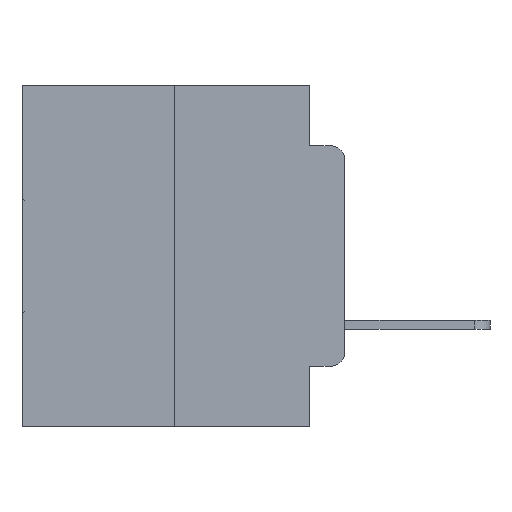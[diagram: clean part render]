
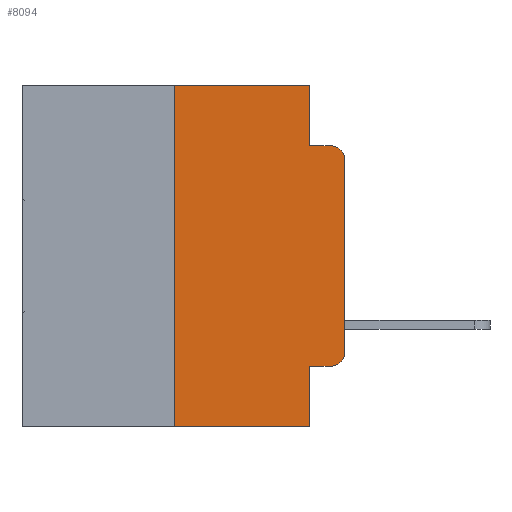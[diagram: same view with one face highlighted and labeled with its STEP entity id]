
A CAD part, left-side view. The second image highlights one B-rep face of the part: STEP entity #8094.
In plain terms, the highlighted planar face has unit normal (-1, 0, 0).
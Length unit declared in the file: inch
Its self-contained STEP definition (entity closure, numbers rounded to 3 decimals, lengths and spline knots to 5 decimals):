
#17 = ORIENTED_EDGE ( 'NONE', *, *, #22822, .F. ) ;
#304 = VERTEX_POINT ( 'NONE', #7070 ) ;
#640 = CARTESIAN_POINT ( 'NONE',  ( 0., 0.051, -0.4115 ) ) ;
#647 = ORIENTED_EDGE ( 'NONE', *, *, #26199, .F. ) ;
#725 = ORIENTED_EDGE ( 'NONE', *, *, #19845, .F. ) ;
#1121 = ORIENTED_EDGE ( 'NONE', *, *, #26100, .T. ) ;
#1159 = ORIENTED_EDGE ( 'NONE', *, *, #24348, .F. ) ;
#1205 = CARTESIAN_POINT ( 'NONE',  ( 0., 0.02, -0.3915 ) ) ;
#1344 = LINE ( 'NONE', #10655, #12297 ) ;
#1798 = DIRECTION ( 'NONE',  ( 0., 0., -1. ) ) ;
#2076 = ORIENTED_EDGE ( 'NONE', *, *, #5487, .T. ) ;
#2151 = CARTESIAN_POINT ( 'NONE',  ( 0., 0.25, 0. ) ) ;
#2738 = CARTESIAN_POINT ( 'NONE',  ( 0., 0.473, 0. ) ) ;
#2911 = EDGE_CURVE ( 'NONE', #21207, #26920, #1344, .T. ) ;
#3239 = ORIENTED_EDGE ( 'NONE', *, *, #10179, .T. ) ;
#3328 = DIRECTION ( 'NONE',  ( 0., -1., 0. ) ) ;
#3773 = DIRECTION ( 'NONE',  ( 0., 0., -1. ) ) ;
#5407 = DIRECTION ( 'NONE',  ( 0., -1., 0. ) ) ;
#5487 = EDGE_CURVE ( 'NONE', #23272, #24393, #9509, .T. ) ;
#6623 = LINE ( 'NONE', #21741, #19017 ) ;
#7070 = CARTESIAN_POINT ( 'NONE',  ( 0., 0.25, 0. ) ) ;
#7142 = ORIENTED_EDGE ( 'NONE', *, *, #21871, .F. ) ;
#8011 = VERTEX_POINT ( 'NONE', #21245 ) ;
#8057 = DIRECTION ( 'NONE',  ( 0., -1., 0. ) ) ;
#8094 = ADVANCED_FACE ( 'NONE', ( #28473 ), #26141, .F. ) ;
#8113 = EDGE_LOOP ( 'NONE', ( #11316, #24000, #7142, #17, #647, #725, #1121, #1159, #2076, #3239 ) ) ;
#8690 = CARTESIAN_POINT ( 'NONE',  ( 0., 0.051, 0. ) ) ;
#8902 = CARTESIAN_POINT ( 'NONE',  ( 0., 0.02, -0.4115 ) ) ;
#9316 = VECTOR ( 'NONE', #15556, 39.37008 ) ;
#9509 = LINE ( 'NONE', #640, #15018 ) ;
#10179 = EDGE_CURVE ( 'NONE', #24393, #21207, #17766, .T. ) ;
#10578 = DIRECTION ( 'NONE',  ( 0., 0., 1. ) ) ;
#10655 = CARTESIAN_POINT ( 'NONE',  ( 0., 0., 0. ) ) ;
#11089 = VERTEX_POINT ( 'NONE', #29963 ) ;
#11316 = ORIENTED_EDGE ( 'NONE', *, *, #2911, .T. ) ;
#12185 = VERTEX_POINT ( 'NONE', #29485 ) ;
#12297 = VECTOR ( 'NONE', #10578, 39.37008 ) ;
#12768 = DIRECTION ( 'NONE',  ( 1., 0., 0. ) ) ;
#13389 = VERTEX_POINT ( 'NONE', #25310 ) ;
#14238 = VECTOR ( 'NONE', #14439, 39.37008 ) ;
#14415 = CARTESIAN_POINT ( 'NONE',  ( 0., 0.051, 0. ) ) ;
#14439 = DIRECTION ( 'NONE',  ( 0., 0., 1. ) ) ;
#14841 = VECTOR ( 'NONE', #3328, 39.37008 ) ;
#15018 = VECTOR ( 'NONE', #5407, 39.37008 ) ;
#15548 = LINE ( 'NONE', #26556, #14841 ) ;
#15556 = DIRECTION ( 'NONE',  ( 0., -1., 0. ) ) ;
#16249 = LINE ( 'NONE', #28699, #9316 ) ;
#16383 = DIRECTION ( 'NONE',  ( -1., 0., 0. ) ) ;
#16714 = DIRECTION ( 'NONE',  ( 0., 0., -1. ) ) ;
#17063 = VERTEX_POINT ( 'NONE', #29218 ) ;
#17766 = CIRCLE ( 'NONE', #21266, 0.02 ) ;
#18097 = DIRECTION ( 'NONE',  ( -1., 0., 0. ) ) ;
#18404 = CARTESIAN_POINT ( 'NONE',  ( 0., 0.051, -0.4115 ) ) ;
#18503 = VECTOR ( 'NONE', #26839, 39.37008 ) ;
#18610 = LINE ( 'NONE', #14415, #24522 ) ;
#19017 = VECTOR ( 'NONE', #8057, 39.37008 ) ;
#19167 = LINE ( 'NONE', #8690, #18503 ) ;
#19631 = CARTESIAN_POINT ( 'NONE',  ( 0., 0., -0.3915 ) ) ;
#19845 = EDGE_CURVE ( 'NONE', #13389, #304, #21520, .T. ) ;
#21207 = VERTEX_POINT ( 'NONE', #19631 ) ;
#21229 = AXIS2_PLACEMENT_3D ( 'NONE', #2738, #12768, #28267 ) ;
#21245 = CARTESIAN_POINT ( 'NONE',  ( 0., 0.051, 0. ) ) ;
#21266 = AXIS2_PLACEMENT_3D ( 'NONE', #1205, #18097, #3773 ) ;
#21520 = LINE ( 'NONE', #2151, #14238 ) ;
#21741 = CARTESIAN_POINT ( 'NONE',  ( 0., 0.473, -0.5 ) ) ;
#21871 = EDGE_CURVE ( 'NONE', #12185, #17063, #16249, .T. ) ;
#22004 = CIRCLE ( 'NONE', #28862, 0.02 ) ;
#22822 = EDGE_CURVE ( 'NONE', #8011, #12185, #18610, .T. ) ;
#23272 = VERTEX_POINT ( 'NONE', #18404 ) ;
#24000 = ORIENTED_EDGE ( 'NONE', *, *, #27814, .T. ) ;
#24348 = EDGE_CURVE ( 'NONE', #23272, #11089, #19167, .T. ) ;
#24393 = VERTEX_POINT ( 'NONE', #8902 ) ;
#24522 = VECTOR ( 'NONE', #16714, 39.37008 ) ;
#25310 = CARTESIAN_POINT ( 'NONE',  ( 0., 0.25, -0.5 ) ) ;
#26100 = EDGE_CURVE ( 'NONE', #13389, #11089, #6623, .T. ) ;
#26141 = PLANE ( 'NONE',  #21229 ) ;
#26199 = EDGE_CURVE ( 'NONE', #304, #8011, #15548, .T. ) ;
#26556 = CARTESIAN_POINT ( 'NONE',  ( 0., 0.473, 0. ) ) ;
#26839 = DIRECTION ( 'NONE',  ( 0., 0., -1. ) ) ;
#26920 = VERTEX_POINT ( 'NONE', #28416 ) ;
#27814 = EDGE_CURVE ( 'NONE', #26920, #17063, #22004, .T. ) ;
#28267 = DIRECTION ( 'NONE',  ( 0., 0., -1. ) ) ;
#28416 = CARTESIAN_POINT ( 'NONE',  ( 0., 0., -0.1085 ) ) ;
#28473 = FACE_OUTER_BOUND ( 'NONE', #8113, .T. ) ;
#28699 = CARTESIAN_POINT ( 'NONE',  ( 0., 0.051, -0.0885 ) ) ;
#28862 = AXIS2_PLACEMENT_3D ( 'NONE', #29435, #16383, #1798 ) ;
#29218 = CARTESIAN_POINT ( 'NONE',  ( 0., 0.02, -0.0885 ) ) ;
#29435 = CARTESIAN_POINT ( 'NONE',  ( 0., 0.02, -0.1085 ) ) ;
#29485 = CARTESIAN_POINT ( 'NONE',  ( 0., 0.051, -0.0885 ) ) ;
#29963 = CARTESIAN_POINT ( 'NONE',  ( 0., 0.051, -0.5 ) ) ;
